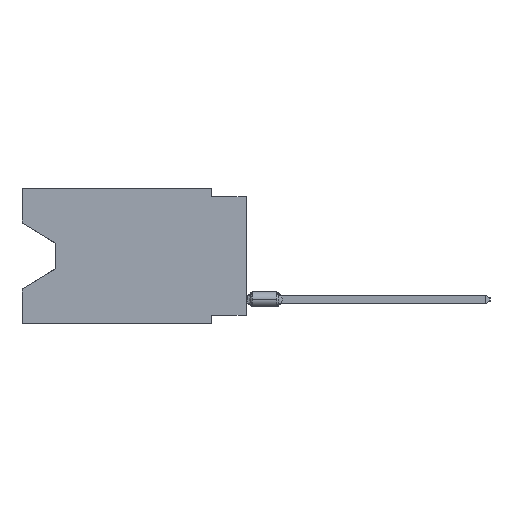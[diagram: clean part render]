
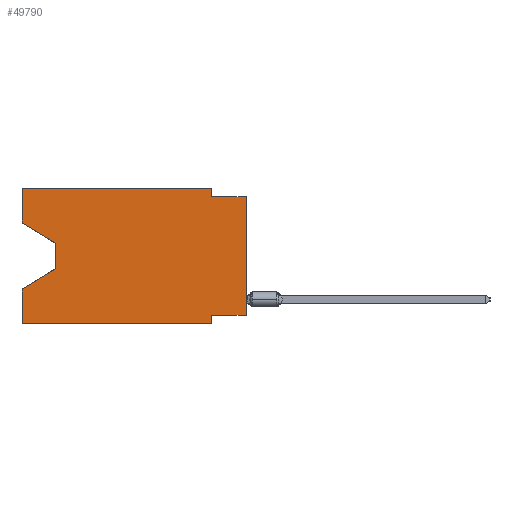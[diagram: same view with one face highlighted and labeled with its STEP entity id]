
A CAD part, left-side view. The second image highlights one B-rep face of the part: STEP entity #49790.
In plain terms, the highlighted planar face has unit normal (-1, 0, 0).
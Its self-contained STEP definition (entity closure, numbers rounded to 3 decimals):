
#531 = ORIENTED_EDGE ( 'NONE', *, *, #23387, .T. ) ;
#737 = DIRECTION ( 'NONE',  ( 0., 0., -1. ) ) ;
#2188 = AXIS2_PLACEMENT_3D ( 'NONE', #33964, #12950, #737 ) ;
#3701 = CARTESIAN_POINT ( 'NONE',  ( 0., 16.383, -9.906 ) ) ;
#3730 = DIRECTION ( 'NONE',  ( 0., 0., 1. ) ) ;
#4192 = VECTOR ( 'NONE', #28207, 1000. ) ;
#4306 = ORIENTED_EDGE ( 'NONE', *, *, #47826, .F. ) ;
#5190 = DIRECTION ( 'NONE',  ( 0., 0., 1. ) ) ;
#5940 = LINE ( 'NONE', #15235, #40566 ) ;
#7552 = VERTEX_POINT ( 'NONE', #25302 ) ;
#8540 = VECTOR ( 'NONE', #5190, 1000. ) ;
#10117 = ORIENTED_EDGE ( 'NONE', *, *, #21479, .F. ) ;
#10252 = LINE ( 'NONE', #23009, #38013 ) ;
#11426 = ORIENTED_EDGE ( 'NONE', *, *, #11608, .F. ) ;
#11438 = LINE ( 'NONE', #44114, #12111 ) ;
#11608 = EDGE_CURVE ( 'NONE', #44805, #7552, #29922, .T. ) ;
#12111 = VECTOR ( 'NONE', #3730, 1000. ) ;
#12554 = LINE ( 'NONE', #17618, #29319 ) ;
#12694 = PLANE ( 'NONE',  #2188 ) ;
#12950 = DIRECTION ( 'NONE',  ( 1., 0., 0. ) ) ;
#13071 = EDGE_CURVE ( 'NONE', #41071, #39287, #11438, .T. ) ;
#13902 = CARTESIAN_POINT ( 'NONE',  ( 0., 2.54, -9.906 ) ) ;
#14585 = DIRECTION ( 'NONE',  ( 0., -0.855, -0.519 ) ) ;
#14653 = CARTESIAN_POINT ( 'NONE',  ( 0., 16.383, 0. ) ) ;
#14678 = VECTOR ( 'NONE', #25790, 1000. ) ;
#14991 = CARTESIAN_POINT ( 'NONE',  ( 0., 16.383, 0. ) ) ;
#15115 = LINE ( 'NONE', #50953, #28914 ) ;
#15235 = CARTESIAN_POINT ( 'NONE',  ( 0., 16.383, -9.906 ) ) ;
#15719 = CARTESIAN_POINT ( 'NONE',  ( 0., 0., -0.635 ) ) ;
#16090 = CARTESIAN_POINT ( 'NONE',  ( 0., 13.97, -4.013 ) ) ;
#16539 = VERTEX_POINT ( 'NONE', #44269 ) ;
#17273 = LINE ( 'NONE', #37475, #14678 ) ;
#17618 = CARTESIAN_POINT ( 'NONE',  ( 0., 16.383, 0. ) ) ;
#18548 = VECTOR ( 'NONE', #47271, 1000. ) ;
#20820 = VECTOR ( 'NONE', #28328, 1000. ) ;
#21479 = EDGE_CURVE ( 'NONE', #51371, #36088, #42050, .T. ) ;
#21514 = ORIENTED_EDGE ( 'NONE', *, *, #24952, .F. ) ;
#22361 = EDGE_CURVE ( 'NONE', #36088, #43266, #47563, .T. ) ;
#22395 = EDGE_CURVE ( 'NONE', #43266, #39287, #43862, .T. ) ;
#23009 = CARTESIAN_POINT ( 'NONE',  ( 0., 13.97, -5.893 ) ) ;
#23387 = EDGE_CURVE ( 'NONE', #34187, #33132, #15115, .T. ) ;
#24952 = EDGE_CURVE ( 'NONE', #41071, #16539, #17273, .T. ) ;
#25302 = CARTESIAN_POINT ( 'NONE',  ( 0., 16.383, -7.36 ) ) ;
#25335 = DIRECTION ( 'NONE',  ( 0., 0., 1. ) ) ;
#25479 = FACE_OUTER_BOUND ( 'NONE', #26674, .T. ) ;
#25787 = ORIENTED_EDGE ( 'NONE', *, *, #13071, .T. ) ;
#25790 = DIRECTION ( 'NONE',  ( 0., 1., 0. ) ) ;
#26201 = CARTESIAN_POINT ( 'NONE',  ( 0., 16.383, 0. ) ) ;
#26674 = EDGE_LOOP ( 'NONE', ( #531, #42794, #51849, #11426, #50280, #47025, #21514, #25787, #44067, #51208, #10117, #4306 ) ) ;
#26865 = LINE ( 'NONE', #43053, #18548 ) ;
#27193 = CARTESIAN_POINT ( 'NONE',  ( 0., 0., -9.271 ) ) ;
#27423 = DIRECTION ( 'NONE',  ( 0., 0., -1. ) ) ;
#28207 = DIRECTION ( 'NONE',  ( 0., -1., 0. ) ) ;
#28328 = DIRECTION ( 'NONE',  ( 0., 0., -1. ) ) ;
#28914 = VECTOR ( 'NONE', #14585, 1000. ) ;
#29319 = VECTOR ( 'NONE', #25335, 1000. ) ;
#29922 = LINE ( 'NONE', #26201, #8540 ) ;
#31004 = EDGE_CURVE ( 'NONE', #44805, #35734, #5940, .T. ) ;
#31469 = DIRECTION ( 'NONE',  ( 0., -1., 0. ) ) ;
#33132 = VERTEX_POINT ( 'NONE', #40788 ) ;
#33964 = CARTESIAN_POINT ( 'NONE',  ( 0., 16.383, 0. ) ) ;
#34187 = VERTEX_POINT ( 'NONE', #42676 ) ;
#35389 = CARTESIAN_POINT ( 'NONE',  ( 0., 2.54, 0. ) ) ;
#35669 = EDGE_CURVE ( 'NONE', #33132, #49257, #52443, .T. ) ;
#35734 = VERTEX_POINT ( 'NONE', #13902 ) ;
#36088 = VERTEX_POINT ( 'NONE', #47476 ) ;
#36986 = CARTESIAN_POINT ( 'NONE',  ( 0., 0., -0.635 ) ) ;
#37475 = CARTESIAN_POINT ( 'NONE',  ( 0., 0., -9.271 ) ) ;
#37640 = EDGE_CURVE ( 'NONE', #49257, #7552, #10252, .T. ) ;
#38013 = VECTOR ( 'NONE', #50601, 1000. ) ;
#39287 = VERTEX_POINT ( 'NONE', #36986 ) ;
#40566 = VECTOR ( 'NONE', #31469, 1000. ) ;
#40788 = CARTESIAN_POINT ( 'NONE',  ( 0., 13.97, -4.013 ) ) ;
#41071 = VERTEX_POINT ( 'NONE', #27193 ) ;
#42050 = LINE ( 'NONE', #14653, #44904 ) ;
#42573 = DIRECTION ( 'NONE',  ( 0., -1., 0. ) ) ;
#42676 = CARTESIAN_POINT ( 'NONE',  ( 0., 16.383, -2.546 ) ) ;
#42794 = ORIENTED_EDGE ( 'NONE', *, *, #35669, .T. ) ;
#43053 = CARTESIAN_POINT ( 'NONE',  ( 0., 2.54, -9.906 ) ) ;
#43266 = VERTEX_POINT ( 'NONE', #45894 ) ;
#43862 = LINE ( 'NONE', #15719, #4192 ) ;
#44067 = ORIENTED_EDGE ( 'NONE', *, *, #22395, .F. ) ;
#44114 = CARTESIAN_POINT ( 'NONE',  ( 0., 0., 0. ) ) ;
#44187 = VECTOR ( 'NONE', #27423, 1000. ) ;
#44269 = CARTESIAN_POINT ( 'NONE',  ( 0., 2.54, -9.271 ) ) ;
#44805 = VERTEX_POINT ( 'NONE', #3701 ) ;
#44904 = VECTOR ( 'NONE', #42573, 1000. ) ;
#45894 = CARTESIAN_POINT ( 'NONE',  ( 0., 2.54, -0.635 ) ) ;
#47025 = ORIENTED_EDGE ( 'NONE', *, *, #50795, .F. ) ;
#47271 = DIRECTION ( 'NONE',  ( 0., 0., -1. ) ) ;
#47476 = CARTESIAN_POINT ( 'NONE',  ( 0., 2.54, 0. ) ) ;
#47563 = LINE ( 'NONE', #35389, #44187 ) ;
#47826 = EDGE_CURVE ( 'NONE', #34187, #51371, #12554, .T. ) ;
#49257 = VERTEX_POINT ( 'NONE', #50784 ) ;
#49790 = ADVANCED_FACE ( 'NONE', ( #25479 ), #12694, .F. ) ;
#50280 = ORIENTED_EDGE ( 'NONE', *, *, #31004, .T. ) ;
#50601 = DIRECTION ( 'NONE',  ( 0., 0.855, -0.519 ) ) ;
#50784 = CARTESIAN_POINT ( 'NONE',  ( 0., 13.97, -5.893 ) ) ;
#50795 = EDGE_CURVE ( 'NONE', #16539, #35734, #26865, .T. ) ;
#50953 = CARTESIAN_POINT ( 'NONE',  ( 0., 16.383, -2.546 ) ) ;
#51208 = ORIENTED_EDGE ( 'NONE', *, *, #22361, .F. ) ;
#51371 = VERTEX_POINT ( 'NONE', #14991 ) ;
#51849 = ORIENTED_EDGE ( 'NONE', *, *, #37640, .T. ) ;
#52443 = LINE ( 'NONE', #16090, #20820 ) ;
